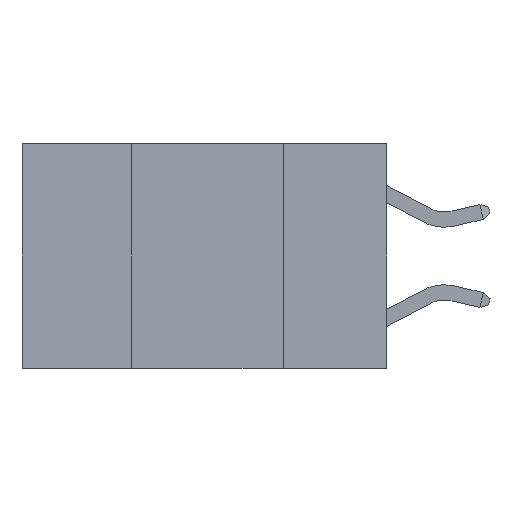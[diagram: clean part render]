
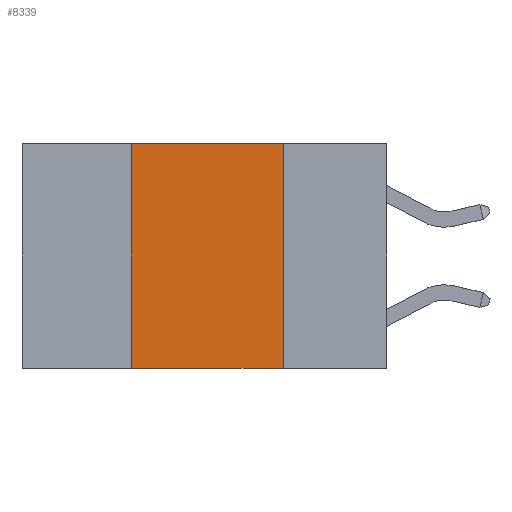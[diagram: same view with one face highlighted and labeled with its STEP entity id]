
A CAD part, left-side view. The second image highlights one B-rep face of the part: STEP entity #8339.
In plain terms, the highlighted planar face has unit normal (-1, 0, 0).
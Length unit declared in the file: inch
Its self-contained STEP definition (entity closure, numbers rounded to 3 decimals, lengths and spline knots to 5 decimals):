
#181 = CARTESIAN_POINT ( 'NONE',  ( 0., 0.42, 0. ) ) ;
#1193 = LINE ( 'NONE', #8440, #2830 ) ;
#1217 = LINE ( 'NONE', #181, #2859 ) ;
#1259 = CARTESIAN_POINT ( 'NONE',  ( 0., 0.6, 0. ) ) ;
#1314 = VERTEX_POINT ( 'NONE', #4251 ) ;
#1630 = EDGE_CURVE ( 'NONE', #1314, #2513, #7457, .T. ) ;
#1929 = LINE ( 'NONE', #3824, #7270 ) ;
#2513 = VERTEX_POINT ( 'NONE', #7828 ) ;
#2531 = CARTESIAN_POINT ( 'NONE',  ( 0., 0.42, -0.37 ) ) ;
#2676 = EDGE_CURVE ( 'NONE', #8262, #6402, #1217, .T. ) ;
#2830 = VECTOR ( 'NONE', #6408, 39.37008 ) ;
#2859 = VECTOR ( 'NONE', #8088, 39.37008 ) ;
#3140 = DIRECTION ( 'NONE',  ( 0., -1., 0. ) ) ;
#3344 = CARTESIAN_POINT ( 'NONE',  ( 0., 0.17, 0. ) ) ;
#3379 = PLANE ( 'NONE',  #5713 ) ;
#3746 = VECTOR ( 'NONE', #5193, 39.37008 ) ;
#3778 = ORIENTED_EDGE ( 'NONE', *, *, #6363, .T. ) ;
#3824 = CARTESIAN_POINT ( 'NONE',  ( 0., 0.6, 0. ) ) ;
#3989 = FACE_OUTER_BOUND ( 'NONE', #7585, .T. ) ;
#4251 = CARTESIAN_POINT ( 'NONE',  ( 0., 0.17, 0. ) ) ;
#4805 = DIRECTION ( 'NONE',  ( 0., 0., -1. ) ) ;
#5193 = DIRECTION ( 'NONE',  ( 0., 0., -1. ) ) ;
#5713 = AXIS2_PLACEMENT_3D ( 'NONE', #1259, #8892, #4805 ) ;
#6363 = EDGE_CURVE ( 'NONE', #8262, #2513, #1193, .T. ) ;
#6402 = VERTEX_POINT ( 'NONE', #7777 ) ;
#6408 = DIRECTION ( 'NONE',  ( 0., -1., 0. ) ) ;
#6557 = ORIENTED_EDGE ( 'NONE', *, *, #2676, .F. ) ;
#7270 = VECTOR ( 'NONE', #3140, 39.37008 ) ;
#7307 = ORIENTED_EDGE ( 'NONE', *, *, #7624, .F. ) ;
#7457 = LINE ( 'NONE', #3344, #3746 ) ;
#7585 = EDGE_LOOP ( 'NONE', ( #7710, #7307, #6557, #3778 ) ) ;
#7624 = EDGE_CURVE ( 'NONE', #6402, #1314, #1929, .T. ) ;
#7710 = ORIENTED_EDGE ( 'NONE', *, *, #1630, .F. ) ;
#7777 = CARTESIAN_POINT ( 'NONE',  ( 0., 0.42, 0. ) ) ;
#7828 = CARTESIAN_POINT ( 'NONE',  ( 0., 0.17, -0.37 ) ) ;
#8088 = DIRECTION ( 'NONE',  ( 0., 0., 1. ) ) ;
#8262 = VERTEX_POINT ( 'NONE', #2531 ) ;
#8339 = ADVANCED_FACE ( 'NONE', ( #3989 ), #3379, .F. ) ;
#8440 = CARTESIAN_POINT ( 'NONE',  ( 0., 0.6, -0.37 ) ) ;
#8892 = DIRECTION ( 'NONE',  ( 1., 0., 0. ) ) ;
